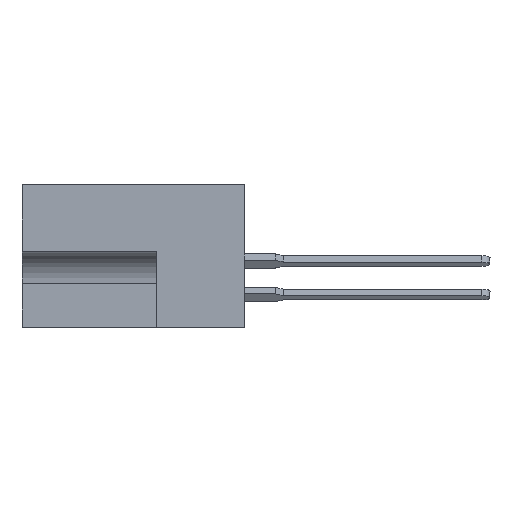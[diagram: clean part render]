
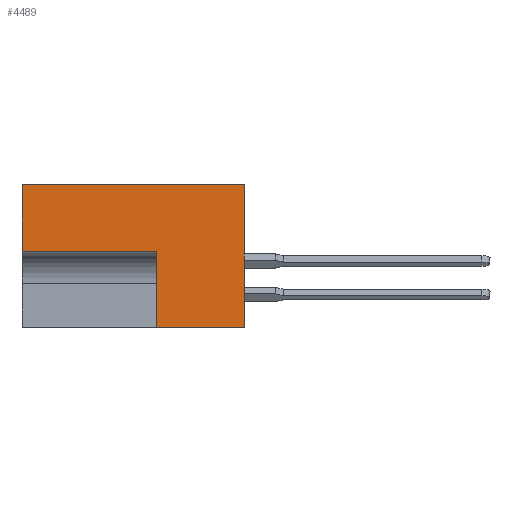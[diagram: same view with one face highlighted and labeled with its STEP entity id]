
A CAD part, left-side view. The second image highlights one B-rep face of the part: STEP entity #4489.
In plain terms, the highlighted planar face has unit normal (-1, 0, 0).
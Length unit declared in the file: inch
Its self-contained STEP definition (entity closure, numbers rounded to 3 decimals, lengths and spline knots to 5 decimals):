
#1095 = CARTESIAN_POINT ( 'NONE',  ( 0., 0.828, 0. ) ) ;
#1117 = VERTEX_POINT ( 'NONE', #19379 ) ;
#1215 = VECTOR ( 'NONE', #13971, 39.37008 ) ;
#1407 = VECTOR ( 'NONE', #13087, 39.37008 ) ;
#1699 = CARTESIAN_POINT ( 'NONE',  ( 0., 0.328, -0.248 ) ) ;
#1810 = VERTEX_POINT ( 'NONE', #6559 ) ;
#2010 = CARTESIAN_POINT ( 'NONE',  ( 0., 0.453, 0. ) ) ;
#2096 = LINE ( 'NONE', #17896, #1407 ) ;
#2352 = LINE ( 'NONE', #2818, #4764 ) ;
#2390 = LINE ( 'NONE', #13463, #16896 ) ;
#2647 = LINE ( 'NONE', #19453, #18824 ) ;
#2744 = DIRECTION ( 'NONE',  ( 0., 0., 1. ) ) ;
#2794 = ORIENTED_EDGE ( 'NONE', *, *, #14408, .F. ) ;
#2818 = CARTESIAN_POINT ( 'NONE',  ( 0., 0.453, -0.531 ) ) ;
#3197 = VERTEX_POINT ( 'NONE', #9920 ) ;
#3294 = CARTESIAN_POINT ( 'NONE',  ( 0., 0.828, 0. ) ) ;
#3339 = VECTOR ( 'NONE', #3485, 39.37008 ) ;
#3485 = DIRECTION ( 'NONE',  ( 0., 0., 1. ) ) ;
#3932 = FACE_OUTER_BOUND ( 'NONE', #7212, .T. ) ;
#4388 = DIRECTION ( 'NONE',  ( 0., -1., 0. ) ) ;
#4489 = ADVANCED_FACE ( 'NONE', ( #3932 ), #8054, .F. ) ;
#4764 = VECTOR ( 'NONE', #19534, 39.37008 ) ;
#6559 = CARTESIAN_POINT ( 'NONE',  ( 0., 0.328, -0.531 ) ) ;
#7212 = EDGE_LOOP ( 'NONE', ( #8756, #15507, #12101, #12417, #18884, #2794 ) ) ;
#7668 = EDGE_CURVE ( 'NONE', #9700, #16492, #7849, .T. ) ;
#7783 = EDGE_CURVE ( 'NONE', #16492, #17213, #11420, .T. ) ;
#7849 = LINE ( 'NONE', #1699, #1215 ) ;
#8054 = PLANE ( 'NONE',  #18468 ) ;
#8756 = ORIENTED_EDGE ( 'NONE', *, *, #7783, .F. ) ;
#9700 = VERTEX_POINT ( 'NONE', #14165 ) ;
#9920 = CARTESIAN_POINT ( 'NONE',  ( 0., 0., -0.531 ) ) ;
#9987 = EDGE_CURVE ( 'NONE', #1810, #3197, #2352, .T. ) ;
#10438 = EDGE_CURVE ( 'NONE', #3197, #1117, #2096, .T. ) ;
#10936 = DIRECTION ( 'NONE',  ( 0., 0., -1. ) ) ;
#11420 = LINE ( 'NONE', #3294, #3339 ) ;
#12101 = ORIENTED_EDGE ( 'NONE', *, *, #19131, .F. ) ;
#12417 = ORIENTED_EDGE ( 'NONE', *, *, #9987, .T. ) ;
#13087 = DIRECTION ( 'NONE',  ( 0., 0., 1. ) ) ;
#13463 = CARTESIAN_POINT ( 'NONE',  ( 0., 0.453, 0. ) ) ;
#13971 = DIRECTION ( 'NONE',  ( 0., 1., 0. ) ) ;
#14165 = CARTESIAN_POINT ( 'NONE',  ( 0., 0.328, -0.248 ) ) ;
#14240 = DIRECTION ( 'NONE',  ( 1., 0., 0. ) ) ;
#14408 = EDGE_CURVE ( 'NONE', #17213, #1117, #2390, .T. ) ;
#15507 = ORIENTED_EDGE ( 'NONE', *, *, #7668, .F. ) ;
#16492 = VERTEX_POINT ( 'NONE', #17249 ) ;
#16896 = VECTOR ( 'NONE', #4388, 39.37008 ) ;
#17213 = VERTEX_POINT ( 'NONE', #1095 ) ;
#17249 = CARTESIAN_POINT ( 'NONE',  ( 0., 0.828, -0.248 ) ) ;
#17896 = CARTESIAN_POINT ( 'NONE',  ( 0., 0., 0. ) ) ;
#18468 = AXIS2_PLACEMENT_3D ( 'NONE', #2010, #14240, #10936 ) ;
#18824 = VECTOR ( 'NONE', #2744, 39.37008 ) ;
#18884 = ORIENTED_EDGE ( 'NONE', *, *, #10438, .T. ) ;
#19131 = EDGE_CURVE ( 'NONE', #1810, #9700, #2647, .T. ) ;
#19379 = CARTESIAN_POINT ( 'NONE',  ( 0., 0., 0. ) ) ;
#19453 = CARTESIAN_POINT ( 'NONE',  ( 0., 0.328, -0.531 ) ) ;
#19534 = DIRECTION ( 'NONE',  ( 0., -1., 0. ) ) ;
